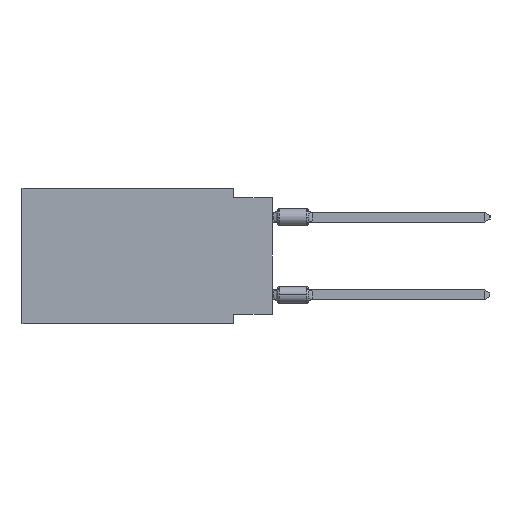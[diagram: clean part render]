
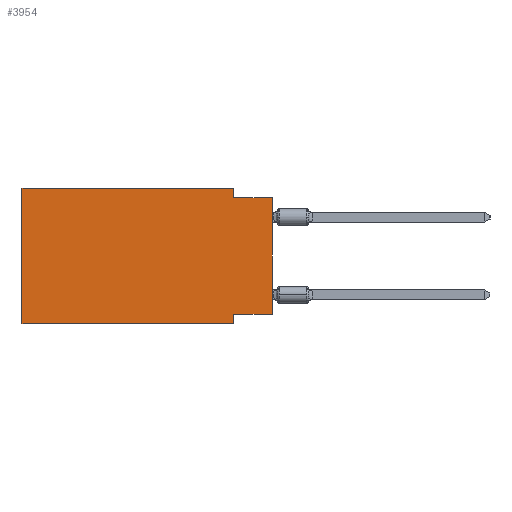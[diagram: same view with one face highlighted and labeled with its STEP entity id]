
A CAD part, left-side view. The second image highlights one B-rep face of the part: STEP entity #3954.
In plain terms, the highlighted planar face has unit normal (-1, 0, 0).
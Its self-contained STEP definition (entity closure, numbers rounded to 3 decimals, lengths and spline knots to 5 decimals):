
#553 = LINE ( 'NONE', #34439, #3135 ) ;
#693 = VERTEX_POINT ( 'NONE', #23578 ) ;
#1577 = CARTESIAN_POINT ( 'NONE',  ( 0., 0.1, -0.35 ) ) ;
#3135 = VECTOR ( 'NONE', #46105, 39.37008 ) ;
#3704 = CARTESIAN_POINT ( 'NONE',  ( 0., 0.645, 0. ) ) ;
#3954 = ADVANCED_FACE ( 'NONE', ( #33322 ), #47577, .F. ) ;
#4081 = CARTESIAN_POINT ( 'NONE',  ( 0., 0.645, -0.35 ) ) ;
#5319 = VECTOR ( 'NONE', #9163, 39.37008 ) ;
#7393 = VERTEX_POINT ( 'NONE', #12428 ) ;
#9060 = EDGE_CURVE ( 'NONE', #19001, #17309, #51597, .T. ) ;
#9163 = DIRECTION ( 'NONE',  ( 0., 0., 1. ) ) ;
#9589 = DIRECTION ( 'NONE',  ( 0., -1., 0. ) ) ;
#10054 = CARTESIAN_POINT ( 'NONE',  ( 0., 0.1, 0. ) ) ;
#10556 = ORIENTED_EDGE ( 'NONE', *, *, #9060, .T. ) ;
#12428 = CARTESIAN_POINT ( 'NONE',  ( 0., 0.1, -0.325 ) ) ;
#16762 = DIRECTION ( 'NONE',  ( 0., -1., 0. ) ) ;
#17026 = LINE ( 'NONE', #60708, #45901 ) ;
#17309 = VERTEX_POINT ( 'NONE', #41689 ) ;
#17343 = VERTEX_POINT ( 'NONE', #3704 ) ;
#18113 = ORIENTED_EDGE ( 'NONE', *, *, #27367, .F. ) ;
#18740 = VERTEX_POINT ( 'NONE', #4081 ) ;
#19001 = VERTEX_POINT ( 'NONE', #60690 ) ;
#19297 = CARTESIAN_POINT ( 'NONE',  ( 0., 0., 0. ) ) ;
#20689 = EDGE_CURVE ( 'NONE', #43731, #693, #62325, .T. ) ;
#20895 = DIRECTION ( 'NONE',  ( 0., 0., -1. ) ) ;
#22357 = CARTESIAN_POINT ( 'NONE',  ( 0., 0.1, 0. ) ) ;
#22635 = VECTOR ( 'NONE', #51323, 39.37008 ) ;
#23450 = EDGE_CURVE ( 'NONE', #17343, #43731, #48231, .T. ) ;
#23578 = CARTESIAN_POINT ( 'NONE',  ( 0., 0.1, -0.025 ) ) ;
#24141 = DIRECTION ( 'NONE',  ( 1., 0., 0. ) ) ;
#25910 = ORIENTED_EDGE ( 'NONE', *, *, #20689, .F. ) ;
#27367 = EDGE_CURVE ( 'NONE', #693, #17309, #553, .T. ) ;
#30892 = ORIENTED_EDGE ( 'NONE', *, *, #32151, .F. ) ;
#32151 = EDGE_CURVE ( 'NONE', #19001, #7393, #61458, .T. ) ;
#32284 = ORIENTED_EDGE ( 'NONE', *, *, #58931, .F. ) ;
#33322 = FACE_OUTER_BOUND ( 'NONE', #42693, .T. ) ;
#33354 = CARTESIAN_POINT ( 'NONE',  ( 0., 0.645, 0. ) ) ;
#34439 = CARTESIAN_POINT ( 'NONE',  ( 0., 0., -0.025 ) ) ;
#35982 = ORIENTED_EDGE ( 'NONE', *, *, #58497, .F. ) ;
#36377 = CARTESIAN_POINT ( 'NONE',  ( 0., 0.645, -0.35 ) ) ;
#38961 = VECTOR ( 'NONE', #16762, 39.37008 ) ;
#39110 = AXIS2_PLACEMENT_3D ( 'NONE', #62464, #24141, #43457 ) ;
#41689 = CARTESIAN_POINT ( 'NONE',  ( 0., 0., -0.025 ) ) ;
#42693 = EDGE_LOOP ( 'NONE', ( #10556, #18113, #25910, #58863, #32284, #52988, #35982, #30892 ) ) ;
#43457 = DIRECTION ( 'NONE',  ( 0., 0., -1. ) ) ;
#43731 = VERTEX_POINT ( 'NONE', #22357 ) ;
#44955 = LINE ( 'NONE', #1577, #62050 ) ;
#45270 = VECTOR ( 'NONE', #9589, 39.37008 ) ;
#45901 = VECTOR ( 'NONE', #60392, 39.37008 ) ;
#46105 = DIRECTION ( 'NONE',  ( 0., -1., 0. ) ) ;
#47577 = PLANE ( 'NONE',  #39110 ) ;
#48123 = VECTOR ( 'NONE', #57569, 39.37008 ) ;
#48231 = LINE ( 'NONE', #33354, #45270 ) ;
#48468 = VERTEX_POINT ( 'NONE', #53405 ) ;
#50628 = LINE ( 'NONE', #36377, #38961 ) ;
#51323 = DIRECTION ( 'NONE',  ( 0., 1., 0. ) ) ;
#51597 = LINE ( 'NONE', #19297, #5319 ) ;
#52988 = ORIENTED_EDGE ( 'NONE', *, *, #60029, .T. ) ;
#53405 = CARTESIAN_POINT ( 'NONE',  ( 0., 0.1, -0.35 ) ) ;
#55456 = CARTESIAN_POINT ( 'NONE',  ( 0., 0., -0.325 ) ) ;
#57569 = DIRECTION ( 'NONE',  ( 0., 0., -1. ) ) ;
#58497 = EDGE_CURVE ( 'NONE', #7393, #48468, #44955, .T. ) ;
#58863 = ORIENTED_EDGE ( 'NONE', *, *, #23450, .F. ) ;
#58931 = EDGE_CURVE ( 'NONE', #18740, #17343, #17026, .T. ) ;
#60029 = EDGE_CURVE ( 'NONE', #18740, #48468, #50628, .T. ) ;
#60392 = DIRECTION ( 'NONE',  ( 0., 0., 1. ) ) ;
#60690 = CARTESIAN_POINT ( 'NONE',  ( 0., 0., -0.325 ) ) ;
#60708 = CARTESIAN_POINT ( 'NONE',  ( 0., 0.645, 0. ) ) ;
#61458 = LINE ( 'NONE', #55456, #22635 ) ;
#62050 = VECTOR ( 'NONE', #20895, 39.37008 ) ;
#62325 = LINE ( 'NONE', #10054, #48123 ) ;
#62464 = CARTESIAN_POINT ( 'NONE',  ( 0., 0.645, 0. ) ) ;
